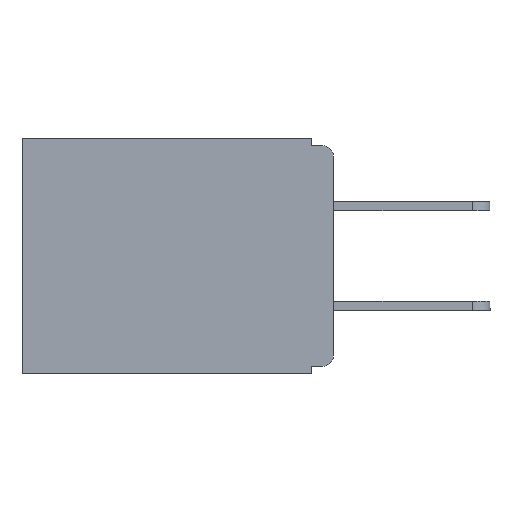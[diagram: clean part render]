
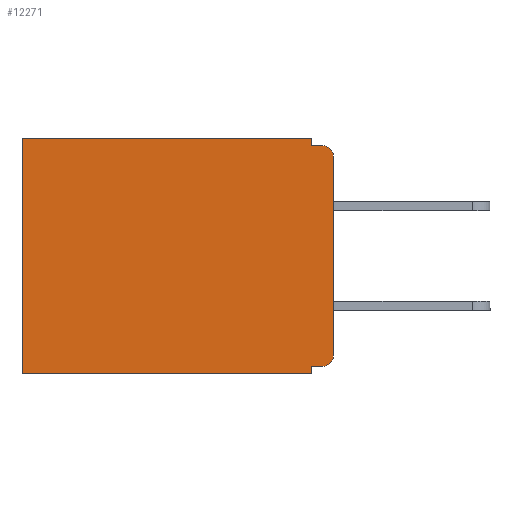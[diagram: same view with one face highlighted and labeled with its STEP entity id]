
A CAD part, left-side view. The second image highlights one B-rep face of the part: STEP entity #12271.
In plain terms, the highlighted planar face has unit normal (-1, 0, 0).
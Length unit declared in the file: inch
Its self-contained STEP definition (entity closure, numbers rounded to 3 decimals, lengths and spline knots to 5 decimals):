
#194 = ORIENTED_EDGE ( 'NONE', *, *, #4831, .F. ) ;
#576 = VECTOR ( 'NONE', #8761, 39.37008 ) ;
#611 = EDGE_CURVE ( 'NONE', #5442, #14948, #4704, .T. ) ;
#910 = CARTESIAN_POINT ( 'NONE',  ( 0.3, 0., -0.33 ) ) ;
#916 = VECTOR ( 'NONE', #2271, 39.37008 ) ;
#1013 = CARTESIAN_POINT ( 'NONE',  ( 0.3, 0.437, -0.33 ) ) ;
#1156 = CARTESIAN_POINT ( 'NONE',  ( 0.3, 0.015, -0.025 ) ) ;
#1197 = EDGE_CURVE ( 'NONE', #2308, #12793, #12644, .T. ) ;
#2107 = PLANE ( 'NONE',  #15473 ) ;
#2271 = DIRECTION ( 'NONE',  ( 0., 1., 0. ) ) ;
#2296 = EDGE_CURVE ( 'NONE', #8512, #5442, #8100, .T. ) ;
#2308 = VERTEX_POINT ( 'NONE', #4898 ) ;
#2351 = CARTESIAN_POINT ( 'NONE',  ( 0.3, 0., -0.32 ) ) ;
#2376 = EDGE_CURVE ( 'NONE', #14475, #5627, #2761, .T. ) ;
#2381 = CARTESIAN_POINT ( 'NONE',  ( 0.3, 0., -0.025 ) ) ;
#2761 = LINE ( 'NONE', #6783, #5761 ) ;
#2795 = ORIENTED_EDGE ( 'NONE', *, *, #14670, .T. ) ;
#2814 = LINE ( 'NONE', #11078, #9503 ) ;
#3087 = LINE ( 'NONE', #2351, #916 ) ;
#3094 = FACE_OUTER_BOUND ( 'NONE', #6467, .T. ) ;
#3139 = CARTESIAN_POINT ( 'NONE',  ( 0.3, 0., -0.305 ) ) ;
#3230 = EDGE_CURVE ( 'NONE', #8151, #5627, #10425, .T. ) ;
#3388 = DIRECTION ( 'NONE',  ( 1., 0., 0. ) ) ;
#4335 = AXIS2_PLACEMENT_3D ( 'NONE', #13713, #9461, #12024 ) ;
#4391 = CARTESIAN_POINT ( 'NONE',  ( 0.3, 0.437, 0. ) ) ;
#4438 = DIRECTION ( 'NONE',  ( 0., -1., 0. ) ) ;
#4616 = ORIENTED_EDGE ( 'NONE', *, *, #7415, .T. ) ;
#4704 = LINE ( 'NONE', #11177, #5106 ) ;
#4809 = ORIENTED_EDGE ( 'NONE', *, *, #1197, .T. ) ;
#4831 = EDGE_CURVE ( 'NONE', #2308, #8512, #3087, .T. ) ;
#4849 = CARTESIAN_POINT ( 'NONE',  ( 0.3, 0.015, -0.01 ) ) ;
#4898 = CARTESIAN_POINT ( 'NONE',  ( 0.3, 0.015, -0.32 ) ) ;
#5106 = VECTOR ( 'NONE', #8596, 39.37008 ) ;
#5442 = VERTEX_POINT ( 'NONE', #11861 ) ;
#5627 = VERTEX_POINT ( 'NONE', #4849 ) ;
#5713 = VERTEX_POINT ( 'NONE', #4391 ) ;
#5761 = VECTOR ( 'NONE', #4438, 39.37008 ) ;
#5989 = DIRECTION ( 'NONE',  ( 0., 0., -1. ) ) ;
#6467 = EDGE_LOOP ( 'NONE', ( #11615, #7339, #9305, #9083, #2795, #4616, #11624, #12826, #194, #4809 ) ) ;
#6783 = CARTESIAN_POINT ( 'NONE',  ( 0.3, 0., -0.01 ) ) ;
#6875 = CARTESIAN_POINT ( 'NONE',  ( 0.3, 0.031, -0.32 ) ) ;
#7339 = ORIENTED_EDGE ( 'NONE', *, *, #3230, .T. ) ;
#7415 = EDGE_CURVE ( 'NONE', #5713, #14948, #11248, .T. ) ;
#8100 = LINE ( 'NONE', #9116, #576 ) ;
#8151 = VERTEX_POINT ( 'NONE', #2381 ) ;
#8412 = DIRECTION ( 'NONE',  ( 0., 0., -1. ) ) ;
#8512 = VERTEX_POINT ( 'NONE', #6875 ) ;
#8555 = DIRECTION ( 'NONE',  ( 0., 0., -1. ) ) ;
#8596 = DIRECTION ( 'NONE',  ( 0., 1., 0. ) ) ;
#8714 = EDGE_CURVE ( 'NONE', #11398, #14475, #2814, .T. ) ;
#8761 = DIRECTION ( 'NONE',  ( 0., 0., -1. ) ) ;
#9083 = ORIENTED_EDGE ( 'NONE', *, *, #8714, .F. ) ;
#9116 = CARTESIAN_POINT ( 'NONE',  ( 0.3, 0.031, -0.33 ) ) ;
#9250 = VECTOR ( 'NONE', #5989, 39.37008 ) ;
#9305 = ORIENTED_EDGE ( 'NONE', *, *, #2376, .F. ) ;
#9461 = DIRECTION ( 'NONE',  ( -1., 0., 0. ) ) ;
#9503 = VECTOR ( 'NONE', #12251, 39.37008 ) ;
#10382 = DIRECTION ( 'NONE',  ( -1., 0., 0. ) ) ;
#10425 = CIRCLE ( 'NONE', #11072, 0.015 ) ;
#10762 = CARTESIAN_POINT ( 'NONE',  ( 0.3, 0., 0. ) ) ;
#10779 = EDGE_CURVE ( 'NONE', #8151, #12793, #15708, .T. ) ;
#10898 = CARTESIAN_POINT ( 'NONE',  ( 0.3, 0., -0.33 ) ) ;
#11072 = AXIS2_PLACEMENT_3D ( 'NONE', #1156, #10382, #8412 ) ;
#11078 = CARTESIAN_POINT ( 'NONE',  ( 0.3, 0.031, 0. ) ) ;
#11177 = CARTESIAN_POINT ( 'NONE',  ( 0.3, 0., -0.33 ) ) ;
#11248 = LINE ( 'NONE', #1013, #14421 ) ;
#11398 = VERTEX_POINT ( 'NONE', #15742 ) ;
#11589 = CARTESIAN_POINT ( 'NONE',  ( 0.3, 0.031, -0.01 ) ) ;
#11615 = ORIENTED_EDGE ( 'NONE', *, *, #10779, .F. ) ;
#11624 = ORIENTED_EDGE ( 'NONE', *, *, #611, .F. ) ;
#11861 = CARTESIAN_POINT ( 'NONE',  ( 0.3, 0.031, -0.33 ) ) ;
#12011 = DIRECTION ( 'NONE',  ( 0., 1., 0. ) ) ;
#12024 = DIRECTION ( 'NONE',  ( 0., 0., -1. ) ) ;
#12135 = DIRECTION ( 'NONE',  ( 0., 0., -1. ) ) ;
#12251 = DIRECTION ( 'NONE',  ( 0., 0., -1. ) ) ;
#12271 = ADVANCED_FACE ( 'NONE', ( #3094 ), #2107, .F. ) ;
#12644 = CIRCLE ( 'NONE', #4335, 0.015 ) ;
#12793 = VERTEX_POINT ( 'NONE', #3139 ) ;
#12826 = ORIENTED_EDGE ( 'NONE', *, *, #2296, .F. ) ;
#13297 = LINE ( 'NONE', #10762, #14591 ) ;
#13713 = CARTESIAN_POINT ( 'NONE',  ( 0.3, 0.015, -0.305 ) ) ;
#14421 = VECTOR ( 'NONE', #8555, 39.37008 ) ;
#14475 = VERTEX_POINT ( 'NONE', #11589 ) ;
#14591 = VECTOR ( 'NONE', #12011, 39.37008 ) ;
#14670 = EDGE_CURVE ( 'NONE', #11398, #5713, #13297, .T. ) ;
#14725 = CARTESIAN_POINT ( 'NONE',  ( 0.3, 0.437, -0.33 ) ) ;
#14948 = VERTEX_POINT ( 'NONE', #14725 ) ;
#15473 = AXIS2_PLACEMENT_3D ( 'NONE', #10898, #3388, #12135 ) ;
#15708 = LINE ( 'NONE', #910, #9250 ) ;
#15742 = CARTESIAN_POINT ( 'NONE',  ( 0.3, 0.031, 0. ) ) ;
